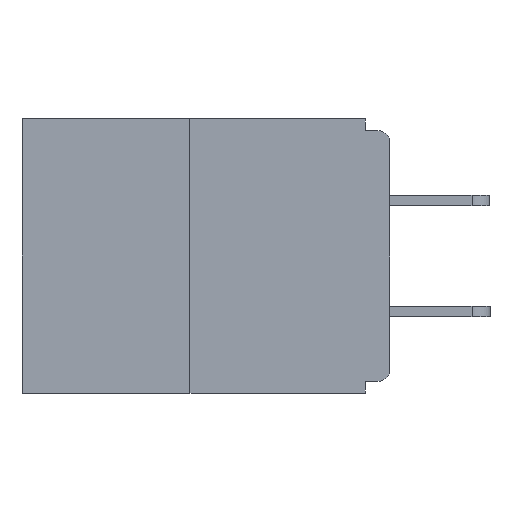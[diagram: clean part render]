
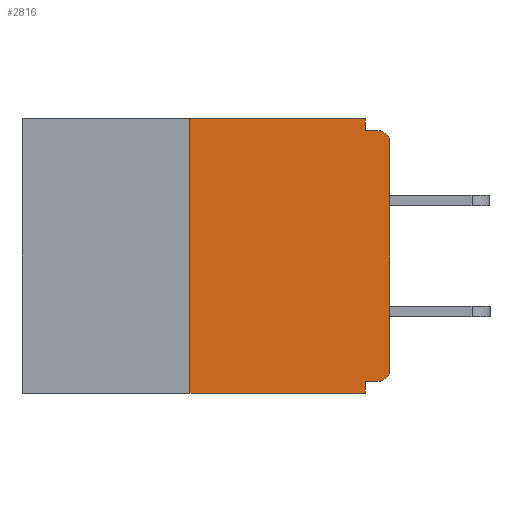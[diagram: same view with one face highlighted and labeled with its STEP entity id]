
A CAD part, left-side view. The second image highlights one B-rep face of the part: STEP entity #2816.
In plain terms, the highlighted planar face has unit normal (-1, 0, 0).
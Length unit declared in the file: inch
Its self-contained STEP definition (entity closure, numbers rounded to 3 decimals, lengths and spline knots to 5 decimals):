
#115 = EDGE_CURVE ( 'NONE', #10172, #6142, #12397, .T. ) ;
#134 = CARTESIAN_POINT ( 'NONE',  ( 0., 0.46, 0. ) ) ;
#199 = CARTESIAN_POINT ( 'NONE',  ( 0., 0.031, -0.328 ) ) ;
#260 = AXIS2_PLACEMENT_3D ( 'NONE', #134, #2170, #9494 ) ;
#455 = CARTESIAN_POINT ( 'NONE',  ( 0., 0.25, 0. ) ) ;
#549 = ORIENTED_EDGE ( 'NONE', *, *, #8560, .F. ) ;
#698 = CARTESIAN_POINT ( 'NONE',  ( 0., 0., -0.313 ) ) ;
#771 = CARTESIAN_POINT ( 'NONE',  ( 0., 0.015, -0.313 ) ) ;
#785 = ORIENTED_EDGE ( 'NONE', *, *, #970, .T. ) ;
#808 = VECTOR ( 'NONE', #11922, 39.37008 ) ;
#970 = EDGE_CURVE ( 'NONE', #8145, #10172, #7892, .T. ) ;
#1004 = LINE ( 'NONE', #10586, #2976 ) ;
#1181 = DIRECTION ( 'NONE',  ( 0., 0., -1. ) ) ;
#1269 = EDGE_CURVE ( 'NONE', #7786, #6142, #1004, .T. ) ;
#1633 = DIRECTION ( 'NONE',  ( -1., 0., 0. ) ) ;
#1667 = VERTEX_POINT ( 'NONE', #455 ) ;
#1669 = VECTOR ( 'NONE', #4199, 39.37008 ) ;
#2063 = VERTEX_POINT ( 'NONE', #12407 ) ;
#2170 = DIRECTION ( 'NONE',  ( 1., 0., 0. ) ) ;
#2258 = DIRECTION ( 'NONE',  ( 0., 0., -1. ) ) ;
#2326 = LINE ( 'NONE', #11889, #13223 ) ;
#2760 = DIRECTION ( 'NONE',  ( 0., 0., 1. ) ) ;
#2772 = ORIENTED_EDGE ( 'NONE', *, *, #10352, .F. ) ;
#2816 = ADVANCED_FACE ( 'NONE', ( #8681 ), #8478, .F. ) ;
#2976 = VECTOR ( 'NONE', #6449, 39.37008 ) ;
#3027 = EDGE_CURVE ( 'NONE', #4672, #1667, #5687, .T. ) ;
#3135 = CARTESIAN_POINT ( 'NONE',  ( 0., 0., -0.03 ) ) ;
#3212 = ORIENTED_EDGE ( 'NONE', *, *, #13437, .F. ) ;
#3561 = VECTOR ( 'NONE', #1181, 39.37008 ) ;
#3569 = LINE ( 'NONE', #6832, #808 ) ;
#4199 = DIRECTION ( 'NONE',  ( 0., -1., 0. ) ) ;
#4256 = AXIS2_PLACEMENT_3D ( 'NONE', #11482, #6087, #5036 ) ;
#4610 = EDGE_CURVE ( 'NONE', #4672, #2063, #3569, .T. ) ;
#4672 = VERTEX_POINT ( 'NONE', #9293 ) ;
#5036 = DIRECTION ( 'NONE',  ( 0., 0., -1. ) ) ;
#5253 = VERTEX_POINT ( 'NONE', #199 ) ;
#5547 = CARTESIAN_POINT ( 'NONE',  ( 0., 0.015, -0.015 ) ) ;
#5646 = CARTESIAN_POINT ( 'NONE',  ( 0., 0.031, -0.015 ) ) ;
#5687 = LINE ( 'NONE', #11399, #12488 ) ;
#6087 = DIRECTION ( 'NONE',  ( -1., 0., 0. ) ) ;
#6142 = VERTEX_POINT ( 'NONE', #5547 ) ;
#6449 = DIRECTION ( 'NONE',  ( 0., -1., 0. ) ) ;
#6832 = CARTESIAN_POINT ( 'NONE',  ( 0., 0.46, -0.343 ) ) ;
#7064 = VECTOR ( 'NONE', #2258, 39.37008 ) ;
#7298 = VERTEX_POINT ( 'NONE', #11931 ) ;
#7512 = ORIENTED_EDGE ( 'NONE', *, *, #13525, .T. ) ;
#7786 = VERTEX_POINT ( 'NONE', #5646 ) ;
#7892 = LINE ( 'NONE', #9986, #11562 ) ;
#8017 = ORIENTED_EDGE ( 'NONE', *, *, #115, .T. ) ;
#8108 = ORIENTED_EDGE ( 'NONE', *, *, #3027, .F. ) ;
#8145 = VERTEX_POINT ( 'NONE', #698 ) ;
#8248 = DIRECTION ( 'NONE',  ( 0., 0., 1. ) ) ;
#8478 = PLANE ( 'NONE',  #260 ) ;
#8560 = EDGE_CURVE ( 'NONE', #11660, #5253, #2326, .T. ) ;
#8588 = EDGE_LOOP ( 'NONE', ( #2772, #8108, #10785, #3212, #549, #7512, #785, #8017, #10135, #10468 ) ) ;
#8641 = DIRECTION ( 'NONE',  ( 0., 1., 0. ) ) ;
#8681 = FACE_OUTER_BOUND ( 'NONE', #8588, .T. ) ;
#8909 = CARTESIAN_POINT ( 'NONE',  ( 0., 0.46, 0. ) ) ;
#9293 = CARTESIAN_POINT ( 'NONE',  ( 0., 0.25, -0.343 ) ) ;
#9335 = LINE ( 'NONE', #10551, #3561 ) ;
#9397 = AXIS2_PLACEMENT_3D ( 'NONE', #771, #1633, #10115 ) ;
#9494 = DIRECTION ( 'NONE',  ( 0., 0., -1. ) ) ;
#9986 = CARTESIAN_POINT ( 'NONE',  ( 0., 0., 0. ) ) ;
#10115 = DIRECTION ( 'NONE',  ( 0., 0., -1. ) ) ;
#10135 = ORIENTED_EDGE ( 'NONE', *, *, #1269, .F. ) ;
#10172 = VERTEX_POINT ( 'NONE', #3135 ) ;
#10352 = EDGE_CURVE ( 'NONE', #1667, #7298, #13564, .T. ) ;
#10468 = ORIENTED_EDGE ( 'NONE', *, *, #11363, .F. ) ;
#10551 = CARTESIAN_POINT ( 'NONE',  ( 0., 0.031, -0.343 ) ) ;
#10586 = CARTESIAN_POINT ( 'NONE',  ( 0., 0., -0.015 ) ) ;
#10785 = ORIENTED_EDGE ( 'NONE', *, *, #4610, .T. ) ;
#11363 = EDGE_CURVE ( 'NONE', #7298, #7786, #12713, .T. ) ;
#11399 = CARTESIAN_POINT ( 'NONE',  ( 0., 0.25, 0. ) ) ;
#11482 = CARTESIAN_POINT ( 'NONE',  ( 0., 0.015, -0.03 ) ) ;
#11562 = VECTOR ( 'NONE', #2760, 39.37008 ) ;
#11660 = VERTEX_POINT ( 'NONE', #12472 ) ;
#11889 = CARTESIAN_POINT ( 'NONE',  ( 0., 0., -0.328 ) ) ;
#11922 = DIRECTION ( 'NONE',  ( 0., -1., 0. ) ) ;
#11931 = CARTESIAN_POINT ( 'NONE',  ( 0., 0.031, 0. ) ) ;
#12397 = CIRCLE ( 'NONE', #4256, 0.015 ) ;
#12407 = CARTESIAN_POINT ( 'NONE',  ( 0., 0.031, -0.343 ) ) ;
#12472 = CARTESIAN_POINT ( 'NONE',  ( 0., 0.015, -0.328 ) ) ;
#12488 = VECTOR ( 'NONE', #8248, 39.37008 ) ;
#12713 = LINE ( 'NONE', #12794, #7064 ) ;
#12794 = CARTESIAN_POINT ( 'NONE',  ( 0., 0.031, 0. ) ) ;
#13223 = VECTOR ( 'NONE', #8641, 39.37008 ) ;
#13437 = EDGE_CURVE ( 'NONE', #5253, #2063, #9335, .T. ) ;
#13473 = CIRCLE ( 'NONE', #9397, 0.015 ) ;
#13525 = EDGE_CURVE ( 'NONE', #11660, #8145, #13473, .T. ) ;
#13564 = LINE ( 'NONE', #8909, #1669 ) ;
